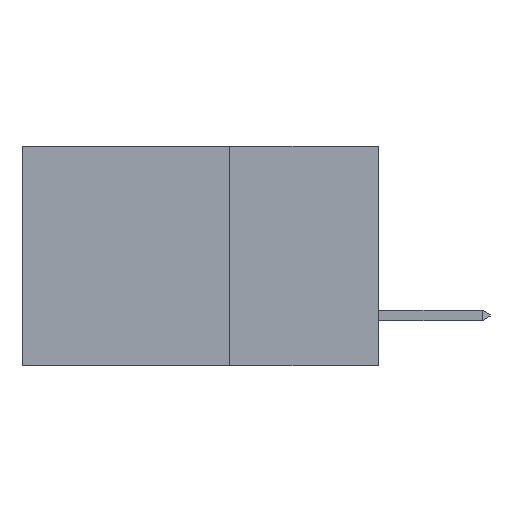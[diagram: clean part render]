
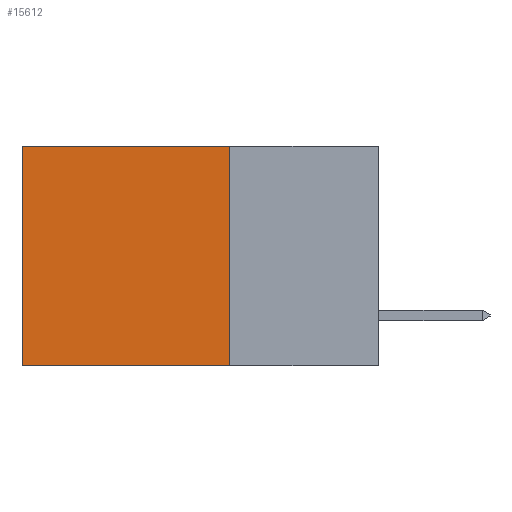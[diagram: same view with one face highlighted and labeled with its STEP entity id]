
A CAD part, left-side view. The second image highlights one B-rep face of the part: STEP entity #15612.
In plain terms, the highlighted planar face has unit normal (-1, 0, 0).
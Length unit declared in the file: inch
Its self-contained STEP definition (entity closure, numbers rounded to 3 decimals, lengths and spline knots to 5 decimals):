
#118 = FACE_OUTER_BOUND ( 'NONE', #6172, .T. ) ;
#1592 = VECTOR ( 'NONE', #7044, 39.37008 ) ;
#1972 = ORIENTED_EDGE ( 'NONE', *, *, #6676, .F. ) ;
#3712 = CARTESIAN_POINT ( 'NONE',  ( 0.298, 0.25, 0. ) ) ;
#4327 = EDGE_CURVE ( 'NONE', #5429, #4652, #6321, .T. ) ;
#4515 = ORIENTED_EDGE ( 'NONE', *, *, #4327, .F. ) ;
#4652 = VERTEX_POINT ( 'NONE', #9134 ) ;
#5035 = CARTESIAN_POINT ( 'NONE',  ( 0.298, 0.25, 0. ) ) ;
#5429 = VERTEX_POINT ( 'NONE', #5035 ) ;
#6172 = EDGE_LOOP ( 'NONE', ( #16080, #1972, #4515, #15817 ) ) ;
#6321 = LINE ( 'NONE', #7681, #1592 ) ;
#6676 = EDGE_CURVE ( 'NONE', #4652, #8008, #10203, .T. ) ;
#7044 = DIRECTION ( 'NONE',  ( 0., 0., -1. ) ) ;
#7681 = CARTESIAN_POINT ( 'NONE',  ( 0.298, 0.25, 0. ) ) ;
#7736 = CARTESIAN_POINT ( 'NONE',  ( 0.298, 0.25, 0. ) ) ;
#8008 = VERTEX_POINT ( 'NONE', #15634 ) ;
#9134 = CARTESIAN_POINT ( 'NONE',  ( 0.298, 0.25, -0.37 ) ) ;
#9360 = DIRECTION ( 'NONE',  ( 1., 0., 0. ) ) ;
#10203 = LINE ( 'NONE', #18734, #17945 ) ;
#12607 = LINE ( 'NONE', #15931, #20249 ) ;
#13360 = VERTEX_POINT ( 'NONE', #15842 ) ;
#13496 = EDGE_CURVE ( 'NONE', #5429, #13360, #15213, .T. ) ;
#14615 = EDGE_CURVE ( 'NONE', #13360, #8008, #12607, .T. ) ;
#15213 = LINE ( 'NONE', #3712, #18855 ) ;
#15612 = ADVANCED_FACE ( 'NONE', ( #118 ), #17068, .F. ) ;
#15634 = CARTESIAN_POINT ( 'NONE',  ( 0.298, 0.6, -0.37 ) ) ;
#15817 = ORIENTED_EDGE ( 'NONE', *, *, #13496, .T. ) ;
#15842 = CARTESIAN_POINT ( 'NONE',  ( 0.298, 0.6, 0. ) ) ;
#15931 = CARTESIAN_POINT ( 'NONE',  ( 0.298, 0.6, 0. ) ) ;
#16080 = ORIENTED_EDGE ( 'NONE', *, *, #14615, .T. ) ;
#17068 = PLANE ( 'NONE',  #19756 ) ;
#17521 = DIRECTION ( 'NONE',  ( 0., 0., -1. ) ) ;
#17837 = DIRECTION ( 'NONE',  ( 0., 1., 0. ) ) ;
#17945 = VECTOR ( 'NONE', #18879, 39.37008 ) ;
#18734 = CARTESIAN_POINT ( 'NONE',  ( 0.298, 0.25, -0.37 ) ) ;
#18855 = VECTOR ( 'NONE', #17837, 39.37008 ) ;
#18879 = DIRECTION ( 'NONE',  ( 0., 1., 0. ) ) ;
#19756 = AXIS2_PLACEMENT_3D ( 'NONE', #7736, #9360, #20183 ) ;
#20183 = DIRECTION ( 'NONE',  ( 0., 0., -1. ) ) ;
#20249 = VECTOR ( 'NONE', #17521, 39.37008 ) ;
